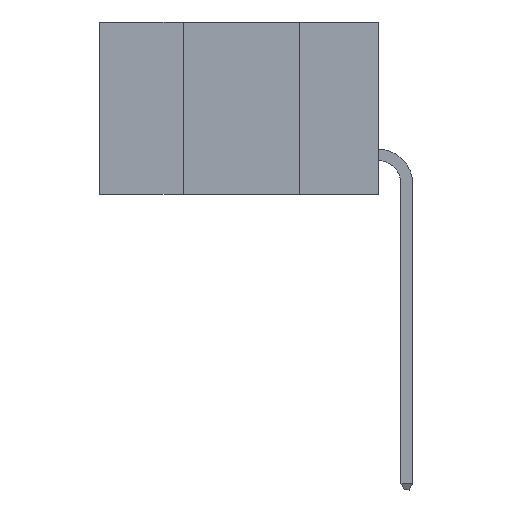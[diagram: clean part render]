
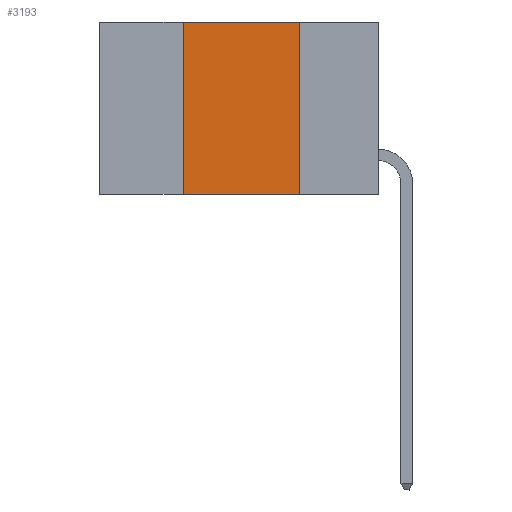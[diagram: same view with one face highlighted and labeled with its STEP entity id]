
A CAD part, left-side view. The second image highlights one B-rep face of the part: STEP entity #3193.
In plain terms, the highlighted planar face has unit normal (-1, 0, 0).
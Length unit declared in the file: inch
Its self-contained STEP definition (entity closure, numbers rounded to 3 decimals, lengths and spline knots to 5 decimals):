
#361 = VECTOR ( 'NONE', #7630, 39.37008 ) ;
#1597 = VERTEX_POINT ( 'NONE', #3625 ) ;
#1910 = EDGE_LOOP ( 'NONE', ( #16426, #5804, #3371, #10968 ) ) ;
#2663 = VERTEX_POINT ( 'NONE', #13999 ) ;
#3193 = ADVANCED_FACE ( 'NONE', ( #5285 ), #16293, .F. ) ;
#3371 = ORIENTED_EDGE ( 'NONE', *, *, #15910, .F. ) ;
#3625 = CARTESIAN_POINT ( 'NONE',  ( 0., 0.42, 0. ) ) ;
#4224 = LINE ( 'NONE', #10445, #361 ) ;
#5170 = LINE ( 'NONE', #15506, #8434 ) ;
#5249 = CARTESIAN_POINT ( 'NONE',  ( 0., 0.6, 0. ) ) ;
#5285 = FACE_OUTER_BOUND ( 'NONE', #1910, .T. ) ;
#5804 = ORIENTED_EDGE ( 'NONE', *, *, #16118, .F. ) ;
#5851 = VERTEX_POINT ( 'NONE', #8807 ) ;
#6854 = DIRECTION ( 'NONE',  ( 0., 0., 1. ) ) ;
#7630 = DIRECTION ( 'NONE',  ( 0., 0., -1. ) ) ;
#8220 = CARTESIAN_POINT ( 'NONE',  ( 0., 0.42, 0. ) ) ;
#8384 = VECTOR ( 'NONE', #14862, 39.37008 ) ;
#8434 = VECTOR ( 'NONE', #16826, 39.37008 ) ;
#8807 = CARTESIAN_POINT ( 'NONE',  ( 0., 0.17, 0. ) ) ;
#9038 = LINE ( 'NONE', #8220, #11867 ) ;
#10445 = CARTESIAN_POINT ( 'NONE',  ( 0., 0.17, 0. ) ) ;
#10968 = ORIENTED_EDGE ( 'NONE', *, *, #14878, .T. ) ;
#11344 = EDGE_CURVE ( 'NONE', #5851, #15236, #4224, .T. ) ;
#11479 = DIRECTION ( 'NONE',  ( 0., 0., -1. ) ) ;
#11562 = DIRECTION ( 'NONE',  ( 1., 0., 0. ) ) ;
#11867 = VECTOR ( 'NONE', #6854, 39.37008 ) ;
#12069 = LINE ( 'NONE', #5249, #8384 ) ;
#13550 = CARTESIAN_POINT ( 'NONE',  ( 0., 0.17, -0.37 ) ) ;
#13999 = CARTESIAN_POINT ( 'NONE',  ( 0., 0.42, -0.37 ) ) ;
#14366 = CARTESIAN_POINT ( 'NONE',  ( 0., 0.6, 0. ) ) ;
#14862 = DIRECTION ( 'NONE',  ( 0., -1., 0. ) ) ;
#14878 = EDGE_CURVE ( 'NONE', #2663, #15236, #5170, .T. ) ;
#15236 = VERTEX_POINT ( 'NONE', #13550 ) ;
#15506 = CARTESIAN_POINT ( 'NONE',  ( 0., 0.6, -0.37 ) ) ;
#15877 = AXIS2_PLACEMENT_3D ( 'NONE', #14366, #11562, #11479 ) ;
#15910 = EDGE_CURVE ( 'NONE', #2663, #1597, #9038, .T. ) ;
#16118 = EDGE_CURVE ( 'NONE', #1597, #5851, #12069, .T. ) ;
#16293 = PLANE ( 'NONE',  #15877 ) ;
#16426 = ORIENTED_EDGE ( 'NONE', *, *, #11344, .F. ) ;
#16826 = DIRECTION ( 'NONE',  ( 0., -1., 0. ) ) ;
